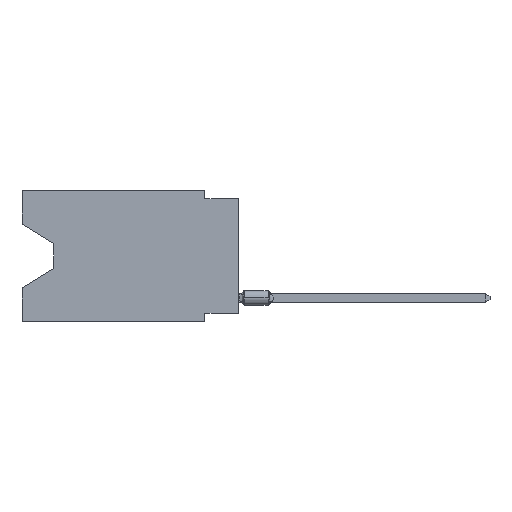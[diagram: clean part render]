
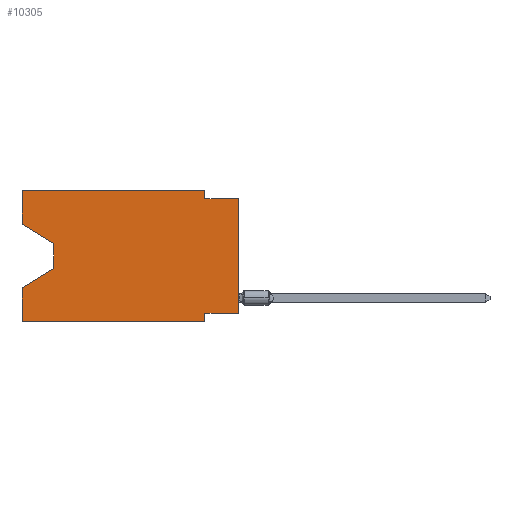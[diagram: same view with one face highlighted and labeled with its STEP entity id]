
A CAD part, left-side view. The second image highlights one B-rep face of the part: STEP entity #10305.
In plain terms, the highlighted planar face has unit normal (-1, 0, 0).
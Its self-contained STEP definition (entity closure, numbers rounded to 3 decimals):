
#153 = ORIENTED_EDGE ( 'NONE', *, *, #7934, .T. ) ;
#541 = VECTOR ( 'NONE', #7500, 1000. ) ;
#808 = VERTEX_POINT ( 'NONE', #2013 ) ;
#845 = VERTEX_POINT ( 'NONE', #13216 ) ;
#1296 = VERTEX_POINT ( 'NONE', #7072 ) ;
#1474 = VECTOR ( 'NONE', #10736, 1000. ) ;
#1511 = ORIENTED_EDGE ( 'NONE', *, *, #4399, .T. ) ;
#1586 = ORIENTED_EDGE ( 'NONE', *, *, #5301, .F. ) ;
#1596 = CARTESIAN_POINT ( 'NONE',  ( 0., 2.54, -9.906 ) ) ;
#1606 = EDGE_CURVE ( 'NONE', #1296, #5689, #12777, .T. ) ;
#1849 = EDGE_CURVE ( 'NONE', #8383, #3922, #13181, .T. ) ;
#1940 = CARTESIAN_POINT ( 'NONE',  ( 0., 0., -0.635 ) ) ;
#2013 = CARTESIAN_POINT ( 'NONE',  ( 0., 13.97, -4.013 ) ) ;
#2055 = LINE ( 'NONE', #5283, #9376 ) ;
#2457 = ORIENTED_EDGE ( 'NONE', *, *, #9957, .F. ) ;
#2560 = VERTEX_POINT ( 'NONE', #7331 ) ;
#2947 = DIRECTION ( 'NONE',  ( 0., 0., -1. ) ) ;
#3036 = ORIENTED_EDGE ( 'NONE', *, *, #7812, .F. ) ;
#3351 = DIRECTION ( 'NONE',  ( 0., 0., 1. ) ) ;
#3489 = DIRECTION ( 'NONE',  ( 0., 0.855, -0.519 ) ) ;
#3495 = DIRECTION ( 'NONE',  ( 0., 0., 1. ) ) ;
#3762 = PLANE ( 'NONE',  #10647 ) ;
#3922 = VERTEX_POINT ( 'NONE', #5894 ) ;
#3949 = CARTESIAN_POINT ( 'NONE',  ( 0., 2.54, 0. ) ) ;
#3992 = CARTESIAN_POINT ( 'NONE',  ( 0., 16.383, 0. ) ) ;
#4060 = LINE ( 'NONE', #10865, #7631 ) ;
#4235 = LINE ( 'NONE', #3949, #7933 ) ;
#4399 = EDGE_CURVE ( 'NONE', #808, #2560, #4060, .T. ) ;
#4768 = VERTEX_POINT ( 'NONE', #9492 ) ;
#4965 = VERTEX_POINT ( 'NONE', #5470 ) ;
#5283 = CARTESIAN_POINT ( 'NONE',  ( 0., 16.383, 0. ) ) ;
#5301 = EDGE_CURVE ( 'NONE', #4768, #4965, #4235, .T. ) ;
#5470 = CARTESIAN_POINT ( 'NONE',  ( 0., 2.54, -0.635 ) ) ;
#5550 = LINE ( 'NONE', #13009, #12270 ) ;
#5689 = VERTEX_POINT ( 'NONE', #1596 ) ;
#5780 = CARTESIAN_POINT ( 'NONE',  ( 0., 16.383, 0. ) ) ;
#5790 = VERTEX_POINT ( 'NONE', #1940 ) ;
#5792 = ORIENTED_EDGE ( 'NONE', *, *, #1849, .F. ) ;
#5886 = CARTESIAN_POINT ( 'NONE',  ( 0., 16.383, -2.546 ) ) ;
#5894 = CARTESIAN_POINT ( 'NONE',  ( 0., 16.383, 0. ) ) ;
#5938 = ORIENTED_EDGE ( 'NONE', *, *, #10883, .F. ) ;
#6099 = EDGE_CURVE ( 'NONE', #8383, #808, #13706, .T. ) ;
#6138 = LINE ( 'NONE', #12750, #541 ) ;
#6163 = VECTOR ( 'NONE', #3495, 1000. ) ;
#6497 = CARTESIAN_POINT ( 'NONE',  ( 0., 16.383, 0. ) ) ;
#6571 = CARTESIAN_POINT ( 'NONE',  ( 0., 13.97, -5.893 ) ) ;
#6792 = DIRECTION ( 'NONE',  ( 1., 0., 0. ) ) ;
#7072 = CARTESIAN_POINT ( 'NONE',  ( 0., 2.54, -9.271 ) ) ;
#7331 = CARTESIAN_POINT ( 'NONE',  ( 0., 13.97, -5.893 ) ) ;
#7386 = CARTESIAN_POINT ( 'NONE',  ( 0., 16.383, -9.906 ) ) ;
#7500 = DIRECTION ( 'NONE',  ( 0., 1., 0. ) ) ;
#7549 = DIRECTION ( 'NONE',  ( 0., -1., 0. ) ) ;
#7574 = DIRECTION ( 'NONE',  ( 0., 0., 1. ) ) ;
#7631 = VECTOR ( 'NONE', #12952, 1000. ) ;
#7787 = LINE ( 'NONE', #6571, #12926 ) ;
#7793 = VECTOR ( 'NONE', #2947, 1000. ) ;
#7812 = EDGE_CURVE ( 'NONE', #13025, #845, #2055, .T. ) ;
#7933 = VECTOR ( 'NONE', #10977, 1000. ) ;
#7934 = EDGE_CURVE ( 'NONE', #10167, #5790, #13100, .T. ) ;
#7936 = ORIENTED_EDGE ( 'NONE', *, *, #10533, .T. ) ;
#7958 = CARTESIAN_POINT ( 'NONE',  ( 0., 0., -0.635 ) ) ;
#8211 = ORIENTED_EDGE ( 'NONE', *, *, #10130, .T. ) ;
#8383 = VERTEX_POINT ( 'NONE', #10937 ) ;
#8793 = CARTESIAN_POINT ( 'NONE',  ( 0., 0., -9.271 ) ) ;
#9171 = ORIENTED_EDGE ( 'NONE', *, *, #6099, .T. ) ;
#9376 = VECTOR ( 'NONE', #7574, 1000. ) ;
#9401 = EDGE_CURVE ( 'NONE', #10167, #1296, #6138, .T. ) ;
#9492 = CARTESIAN_POINT ( 'NONE',  ( 0., 2.54, 0. ) ) ;
#9622 = CARTESIAN_POINT ( 'NONE',  ( 0., 2.54, -9.906 ) ) ;
#9824 = DIRECTION ( 'NONE',  ( 0., -1., 0. ) ) ;
#9957 = EDGE_CURVE ( 'NONE', #3922, #4768, #10461, .T. ) ;
#10060 = ORIENTED_EDGE ( 'NONE', *, *, #1606, .F. ) ;
#10130 = EDGE_CURVE ( 'NONE', #2560, #845, #7787, .T. ) ;
#10167 = VERTEX_POINT ( 'NONE', #8793 ) ;
#10305 = ADVANCED_FACE ( 'NONE', ( #12453 ), #3762, .F. ) ;
#10461 = LINE ( 'NONE', #3992, #1474 ) ;
#10533 = EDGE_CURVE ( 'NONE', #13025, #5689, #5550, .T. ) ;
#10539 = DIRECTION ( 'NONE',  ( 0., -0.855, -0.519 ) ) ;
#10647 = AXIS2_PLACEMENT_3D ( 'NONE', #5780, #6792, #13391 ) ;
#10736 = DIRECTION ( 'NONE',  ( 0., -1., 0. ) ) ;
#10865 = CARTESIAN_POINT ( 'NONE',  ( 0., 13.97, -4.013 ) ) ;
#10883 = EDGE_CURVE ( 'NONE', #4965, #5790, #13413, .T. ) ;
#10937 = CARTESIAN_POINT ( 'NONE',  ( 0., 16.383, -2.546 ) ) ;
#10977 = DIRECTION ( 'NONE',  ( 0., 0., -1. ) ) ;
#12270 = VECTOR ( 'NONE', #7549, 1000. ) ;
#12453 = FACE_OUTER_BOUND ( 'NONE', #13775, .T. ) ;
#12501 = ORIENTED_EDGE ( 'NONE', *, *, #9401, .F. ) ;
#12750 = CARTESIAN_POINT ( 'NONE',  ( 0., 0., -9.271 ) ) ;
#12777 = LINE ( 'NONE', #9622, #7793 ) ;
#12926 = VECTOR ( 'NONE', #3489, 1000. ) ;
#12952 = DIRECTION ( 'NONE',  ( 0., 0., -1. ) ) ;
#13009 = CARTESIAN_POINT ( 'NONE',  ( 0., 16.383, -9.906 ) ) ;
#13025 = VERTEX_POINT ( 'NONE', #7386 ) ;
#13100 = LINE ( 'NONE', #13324, #6163 ) ;
#13179 = VECTOR ( 'NONE', #9824, 1000. ) ;
#13181 = LINE ( 'NONE', #6497, #13764 ) ;
#13216 = CARTESIAN_POINT ( 'NONE',  ( 0., 16.383, -7.36 ) ) ;
#13324 = CARTESIAN_POINT ( 'NONE',  ( 0., 0., 0. ) ) ;
#13391 = DIRECTION ( 'NONE',  ( 0., 0., -1. ) ) ;
#13413 = LINE ( 'NONE', #7958, #13179 ) ;
#13706 = LINE ( 'NONE', #5886, #14060 ) ;
#13764 = VECTOR ( 'NONE', #3351, 1000. ) ;
#13775 = EDGE_LOOP ( 'NONE', ( #9171, #1511, #8211, #3036, #7936, #10060, #12501, #153, #5938, #1586, #2457, #5792 ) ) ;
#14060 = VECTOR ( 'NONE', #10539, 1000. ) ;
